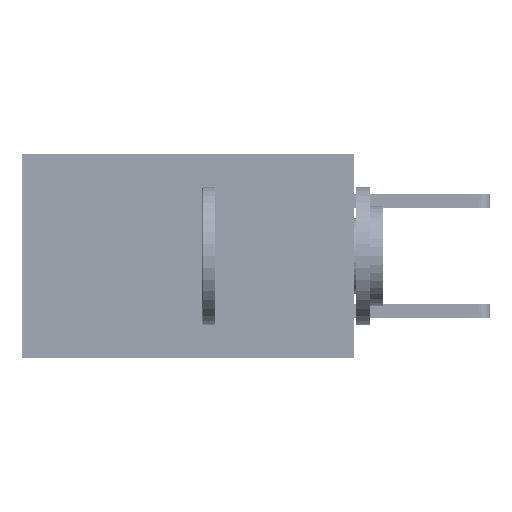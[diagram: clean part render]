
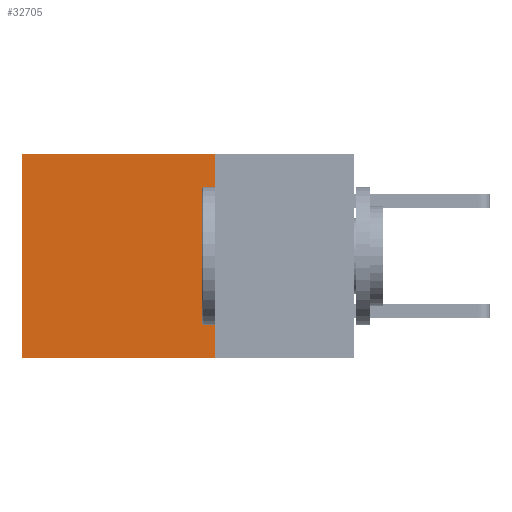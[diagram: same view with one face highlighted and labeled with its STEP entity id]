
A CAD part, left-side view. The second image highlights one B-rep face of the part: STEP entity #32705.
In plain terms, the highlighted planar face has unit normal (-1, 0, 0).
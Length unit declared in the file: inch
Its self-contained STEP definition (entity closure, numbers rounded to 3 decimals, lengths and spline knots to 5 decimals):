
#520 = ORIENTED_EDGE ( 'NONE', *, *, #40921, .T. ) ;
#1386 = VECTOR ( 'NONE', #1910, 39.37008 ) ;
#1707 = DIRECTION ( 'NONE',  ( 1., 0., 0. ) ) ;
#1910 = DIRECTION ( 'NONE',  ( 0., 1., 0. ) ) ;
#2941 = FACE_OUTER_BOUND ( 'NONE', #5296, .T. ) ;
#3478 = CARTESIAN_POINT ( 'NONE',  ( 0.2875, 0.25, -0.37 ) ) ;
#3626 = ORIENTED_EDGE ( 'NONE', *, *, #32043, .T. ) ;
#4816 = VERTEX_POINT ( 'NONE', #32915 ) ;
#5296 = EDGE_LOOP ( 'NONE', ( #520, #33651, #31663, #3626 ) ) ;
#6800 = DIRECTION ( 'NONE',  ( 0., 1., 0. ) ) ;
#7947 = LINE ( 'NONE', #29365, #45148 ) ;
#8194 = EDGE_CURVE ( 'NONE', #25379, #33716, #10218, .T. ) ;
#10218 = LINE ( 'NONE', #34267, #28816 ) ;
#12374 = AXIS2_PLACEMENT_3D ( 'NONE', #22759, #1707, #26249 ) ;
#12811 = CARTESIAN_POINT ( 'NONE',  ( 0.2875, 0.6, 0. ) ) ;
#13355 = DIRECTION ( 'NONE',  ( 0., 0., -1. ) ) ;
#17221 = CARTESIAN_POINT ( 'NONE',  ( 0.2875, 0.25, -0.37 ) ) ;
#18978 = CARTESIAN_POINT ( 'NONE',  ( 0.2875, 0.25, 0. ) ) ;
#22759 = CARTESIAN_POINT ( 'NONE',  ( 0.2875, 0.25, 0. ) ) ;
#25379 = VERTEX_POINT ( 'NONE', #18978 ) ;
#26249 = DIRECTION ( 'NONE',  ( 0., 0., -1. ) ) ;
#26604 = VECTOR ( 'NONE', #6800, 39.37008 ) ;
#27682 = LINE ( 'NONE', #17221, #26604 ) ;
#28816 = VECTOR ( 'NONE', #13355, 39.37008 ) ;
#29365 = CARTESIAN_POINT ( 'NONE',  ( 0.2875, 0.6, 0. ) ) ;
#31663 = ORIENTED_EDGE ( 'NONE', *, *, #8194, .F. ) ;
#32043 = EDGE_CURVE ( 'NONE', #25379, #38261, #39656, .T. ) ;
#32306 = EDGE_CURVE ( 'NONE', #33716, #4816, #27682, .T. ) ;
#32683 = DIRECTION ( 'NONE',  ( 0., 0., -1. ) ) ;
#32705 = ADVANCED_FACE ( 'NONE', ( #2941 ), #36522, .F. ) ;
#32915 = CARTESIAN_POINT ( 'NONE',  ( 0.2875, 0.6, -0.37 ) ) ;
#33651 = ORIENTED_EDGE ( 'NONE', *, *, #32306, .F. ) ;
#33716 = VERTEX_POINT ( 'NONE', #3478 ) ;
#34267 = CARTESIAN_POINT ( 'NONE',  ( 0.2875, 0.25, 0. ) ) ;
#36522 = PLANE ( 'NONE',  #12374 ) ;
#38261 = VERTEX_POINT ( 'NONE', #12811 ) ;
#39656 = LINE ( 'NONE', #43761, #1386 ) ;
#40921 = EDGE_CURVE ( 'NONE', #38261, #4816, #7947, .T. ) ;
#43761 = CARTESIAN_POINT ( 'NONE',  ( 0.2875, 0.25, 0. ) ) ;
#45148 = VECTOR ( 'NONE', #32683, 39.37008 ) ;
